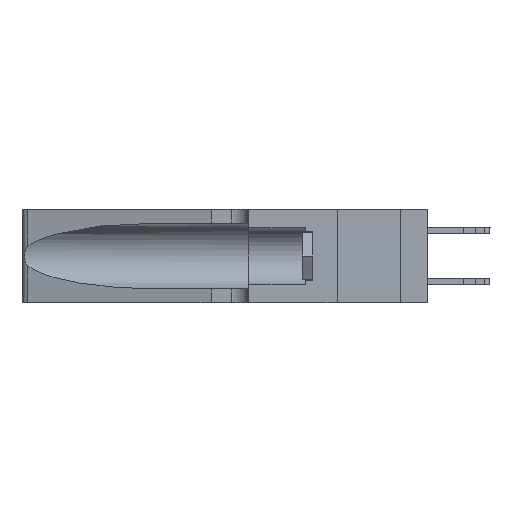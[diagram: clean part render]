
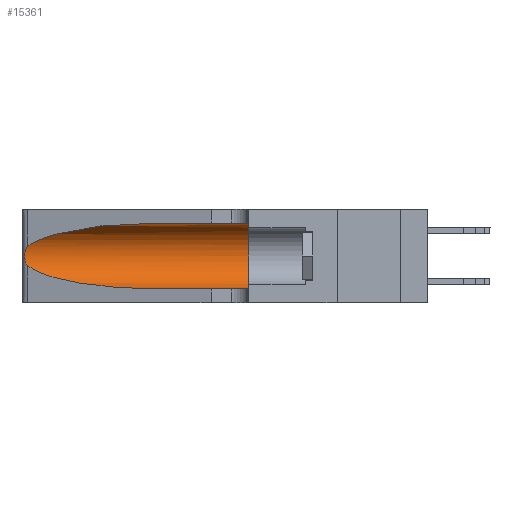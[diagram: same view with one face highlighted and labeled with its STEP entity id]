
A CAD part, left-side view. The second image highlights one B-rep face of the part: STEP entity #15361.
In plain terms, the highlighted cylindrical face has radius 3.308 mm (diameter 6.617 mm), a partial arc.
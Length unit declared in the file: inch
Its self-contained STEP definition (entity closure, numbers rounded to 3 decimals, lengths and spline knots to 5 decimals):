
#328 = EDGE_LOOP ( 'NONE', ( #7910, #12181, #1970, #10094, #9231, #9485 ) ) ;
#415 = EDGE_CURVE ( 'NONE', #13034, #2737, #6393, .T. ) ;
#519 = VERTEX_POINT ( 'NONE', #20000 ) ;
#776 =( BOUNDED_CURVE ( )  B_SPLINE_CURVE ( 3, ( #12058, #18582, #887, #12128 ),
 .UNSPECIFIED., .F., .F. ) 
 B_SPLINE_CURVE_WITH_KNOTS ( ( 4, 4 ),
 ( 1.5708, 2.84003 ),
 .UNSPECIFIED. ) 
 CURVE ( )  GEOMETRIC_REPRESENTATION_ITEM ( )  RATIONAL_B_SPLINE_CURVE ( ( 1., 0.87, 0.87, 1. ) ) 
 REPRESENTATION_ITEM ( '' )  );
#791 = CARTESIAN_POINT ( 'NONE',  ( 0.25555, 1.22994, 0.2215 ) ) ;
#887 = CARTESIAN_POINT ( 'NONE',  ( 0.2373, 1.15595, 0.28018 ) ) ;
#1970 = ORIENTED_EDGE ( 'NONE', *, *, #19813, .T. ) ;
#1978 = AXIS2_PLACEMENT_3D ( 'NONE', #4483, #6171, #20767 ) ;
#2699 = CARTESIAN_POINT ( 'NONE',  ( 0.26075, 1.23896, 0.178 ) ) ;
#2737 = VERTEX_POINT ( 'NONE', #10562 ) ;
#3385 = CARTESIAN_POINT ( 'NONE',  ( 0.18966, 0.96281, 0.05475 ) ) ;
#3403 = CARTESIAN_POINT ( 'NONE',  ( 0.25487, 1.22718, 0.14631 ) ) ;
#3524 = CARTESIAN_POINT ( 'NONE',  ( 0.25487, 1.22718, 0.22369 ) ) ;
#3616 = DIRECTION ( 'NONE',  ( 0., -1., 0. ) ) ;
#3987 = CARTESIAN_POINT ( 'NONE',  ( 0.25639, 1.23184, 0.21858 ) ) ;
#4058 = CARTESIAN_POINT ( 'NONE',  ( 0.26075, 1.23896, 0.19203 ) ) ;
#4227 = CARTESIAN_POINT ( 'NONE',  ( 0.1305, 0.72297, 0.31525 ) ) ;
#4281 = EDGE_CURVE ( 'NONE', #9341, #2737, #18969, .T. ) ;
#4373 = LINE ( 'NONE', #13920, #5867 ) ;
#4483 = CARTESIAN_POINT ( 'NONE',  ( 0.1305, 0.35, 0.185 ) ) ;
#4789 = CARTESIAN_POINT ( 'NONE',  ( 0.1305, 1.61858, 0.185 ) ) ;
#5752 = VERTEX_POINT ( 'NONE', #4227 ) ;
#5867 = VECTOR ( 'NONE', #9679, 39.37008 ) ;
#6171 = DIRECTION ( 'NONE',  ( 0., 1., 0. ) ) ;
#6393 = LINE ( 'NONE', #8527, #19333 ) ;
#6463 = CARTESIAN_POINT ( 'NONE',  ( 0.25639, 1.23186, 0.15144 ) ) ;
#6654 = CARTESIAN_POINT ( 'NONE',  ( 0.1305, 0.72297, 0.05475 ) ) ;
#7910 = ORIENTED_EDGE ( 'NONE', *, *, #12677, .T. ) ;
#8527 = CARTESIAN_POINT ( 'NONE',  ( 0.1305, 1.61858, 0.05475 ) ) ;
#8808 = CARTESIAN_POINT ( 'NONE',  ( 0.1305, 0.72297, 0.05475 ) ) ;
#9231 = ORIENTED_EDGE ( 'NONE', *, *, #4281, .F. ) ;
#9288 = AXIS2_PLACEMENT_3D ( 'NONE', #4789, #12745, #11426 ) ;
#9341 = VERTEX_POINT ( 'NONE', #13919 ) ;
#9485 = ORIENTED_EDGE ( 'NONE', *, *, #14143, .F. ) ;
#9679 = DIRECTION ( 'NONE',  ( 0., -1., 0. ) ) ;
#9993 = CARTESIAN_POINT ( 'NONE',  ( 0.25555, 1.22993, 0.14849 ) ) ;
#10094 = ORIENTED_EDGE ( 'NONE', *, *, #415, .T. ) ;
#10100 = CARTESIAN_POINT ( 'NONE',  ( 0.25787, 1.23484, 0.2124 ) ) ;
#10562 = CARTESIAN_POINT ( 'NONE',  ( 0.1305, 0.35, 0.05475 ) ) ;
#10702 = B_SPLINE_CURVE_WITH_KNOTS ( 'NONE', 3,
 ( #19619, #791, #3987, #10100, #13713, #17130, #4058, #2699, #15441, #17055, #19045, #6463, #9993, #3403 ),
 .UNSPECIFIED., .F., .F.,
 ( 4, 2, 2, 2, 2, 2, 4 ),
 ( 0., 0.00027, 0.00053, 0.00107, 0.0016, 0.00187, 0.00214 ),
 .UNSPECIFIED. ) ;
#11393 = FACE_OUTER_BOUND ( 'NONE', #328, .T. ) ;
#11426 = DIRECTION ( 'NONE',  ( 0., 0., -1. ) ) ;
#11715 =( BOUNDED_CURVE ( )  B_SPLINE_CURVE ( 3, ( #14858, #13245, #3385, #6654 ),
 .UNSPECIFIED., .F., .F. ) 
 B_SPLINE_CURVE_WITH_KNOTS ( ( 4, 4 ),
 ( 3.44316, 4.71239 ),
 .UNSPECIFIED. ) 
 CURVE ( )  GEOMETRIC_REPRESENTATION_ITEM ( )  RATIONAL_B_SPLINE_CURVE ( ( 1., 0.87, 0.87, 1. ) ) 
 REPRESENTATION_ITEM ( '' )  );
#12058 = CARTESIAN_POINT ( 'NONE',  ( 0.1305, 0.72297, 0.31525 ) ) ;
#12128 = CARTESIAN_POINT ( 'NONE',  ( 0.25487, 1.22718, 0.22369 ) ) ;
#12181 = ORIENTED_EDGE ( 'NONE', *, *, #12564, .T. ) ;
#12564 = EDGE_CURVE ( 'NONE', #16661, #519, #10702, .T. ) ;
#12677 = EDGE_CURVE ( 'NONE', #5752, #16661, #776, .T. ) ;
#12745 = DIRECTION ( 'NONE',  ( 0., -1., 0. ) ) ;
#13034 = VERTEX_POINT ( 'NONE', #8808 ) ;
#13245 = CARTESIAN_POINT ( 'NONE',  ( 0.2373, 1.15595, 0.08982 ) ) ;
#13713 = CARTESIAN_POINT ( 'NONE',  ( 0.25854, 1.2359, 0.20912 ) ) ;
#13919 = CARTESIAN_POINT ( 'NONE',  ( 0.1305, 0.35, 0.31525 ) ) ;
#13920 = CARTESIAN_POINT ( 'NONE',  ( 0.1305, 1.61858, 0.31525 ) ) ;
#14143 = EDGE_CURVE ( 'NONE', #5752, #9341, #4373, .T. ) ;
#14662 = CYLINDRICAL_SURFACE ( 'NONE', #9288, 0.13025 ) ;
#14858 = CARTESIAN_POINT ( 'NONE',  ( 0.25487, 1.22718, 0.14631 ) ) ;
#15361 = ADVANCED_FACE ( 'NONE', ( #11393 ), #14662, .F. ) ;
#15441 = CARTESIAN_POINT ( 'NONE',  ( 0.26017, 1.23833, 0.17102 ) ) ;
#16661 = VERTEX_POINT ( 'NONE', #3524 ) ;
#17055 = CARTESIAN_POINT ( 'NONE',  ( 0.25856, 1.23593, 0.16098 ) ) ;
#17130 = CARTESIAN_POINT ( 'NONE',  ( 0.26018, 1.23835, 0.19895 ) ) ;
#18582 = CARTESIAN_POINT ( 'NONE',  ( 0.18966, 0.96281, 0.31525 ) ) ;
#18969 = CIRCLE ( 'NONE', #1978, 0.13025 ) ;
#19045 = CARTESIAN_POINT ( 'NONE',  ( 0.25789, 1.23486, 0.15765 ) ) ;
#19333 = VECTOR ( 'NONE', #3616, 39.37008 ) ;
#19619 = CARTESIAN_POINT ( 'NONE',  ( 0.25487, 1.22718, 0.22369 ) ) ;
#19813 = EDGE_CURVE ( 'NONE', #519, #13034, #11715, .T. ) ;
#20000 = CARTESIAN_POINT ( 'NONE',  ( 0.25487, 1.22718, 0.14631 ) ) ;
#20767 = DIRECTION ( 'NONE',  ( 0., 0., 1. ) ) ;
